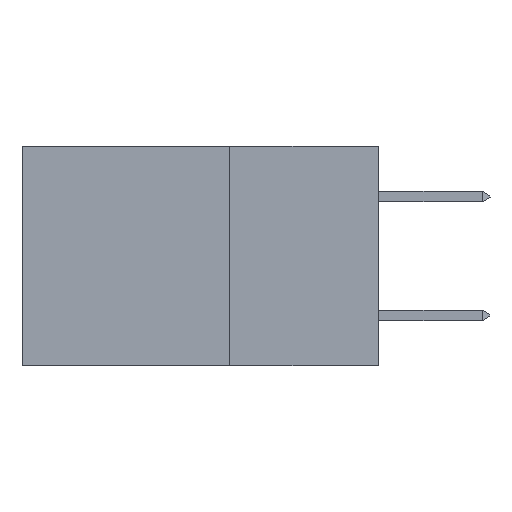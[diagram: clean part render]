
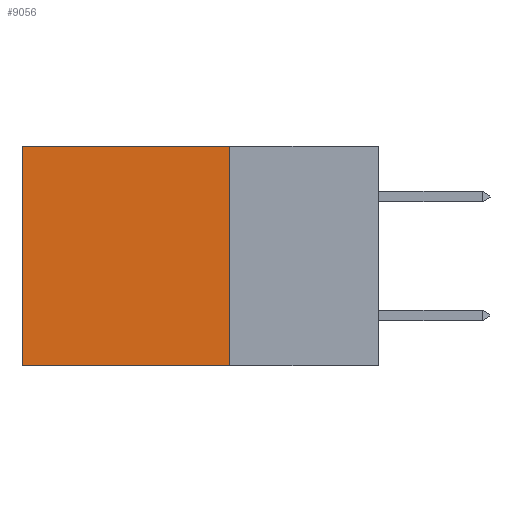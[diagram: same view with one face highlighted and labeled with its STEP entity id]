
A CAD part, left-side view. The second image highlights one B-rep face of the part: STEP entity #9056.
In plain terms, the highlighted planar face has unit normal (-1, 0, 0).
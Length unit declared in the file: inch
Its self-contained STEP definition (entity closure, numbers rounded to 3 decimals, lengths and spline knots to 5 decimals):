
#375 = VERTEX_POINT ( 'NONE', #10993 ) ;
#681 = FACE_OUTER_BOUND ( 'NONE', #2294, .T. ) ;
#1014 = DIRECTION ( 'NONE',  ( 0., 0., -1. ) ) ;
#1057 = VECTOR ( 'NONE', #5978, 39.37008 ) ;
#1110 = ORIENTED_EDGE ( 'NONE', *, *, #8985, .T. ) ;
#1359 = EDGE_CURVE ( 'NONE', #3511, #13293, #1932, .T. ) ;
#1932 = LINE ( 'NONE', #5883, #13370 ) ;
#2178 = CARTESIAN_POINT ( 'NONE',  ( 0.298, 0.6, 0. ) ) ;
#2294 = EDGE_LOOP ( 'NONE', ( #1110, #9230, #5053, #6256 ) ) ;
#3511 = VERTEX_POINT ( 'NONE', #7543 ) ;
#3618 = DIRECTION ( 'NONE',  ( 0., 1., 0. ) ) ;
#5053 = ORIENTED_EDGE ( 'NONE', *, *, #6293, .F. ) ;
#5085 = AXIS2_PLACEMENT_3D ( 'NONE', #14174, #11958, #6084 ) ;
#5883 = CARTESIAN_POINT ( 'NONE',  ( 0.298, 0.25, 0. ) ) ;
#5978 = DIRECTION ( 'NONE',  ( 0., 0., -1. ) ) ;
#6017 = DIRECTION ( 'NONE',  ( 0., 1., 0. ) ) ;
#6084 = DIRECTION ( 'NONE',  ( 0., 0., -1. ) ) ;
#6256 = ORIENTED_EDGE ( 'NONE', *, *, #1359, .T. ) ;
#6293 = EDGE_CURVE ( 'NONE', #3511, #375, #9834, .T. ) ;
#7166 = CARTESIAN_POINT ( 'NONE',  ( 0.298, 0.25, -0.37 ) ) ;
#7177 = PLANE ( 'NONE',  #5085 ) ;
#7543 = CARTESIAN_POINT ( 'NONE',  ( 0.298, 0.25, 0. ) ) ;
#7818 = CARTESIAN_POINT ( 'NONE',  ( 0.298, 0.6, 0. ) ) ;
#8434 = VECTOR ( 'NONE', #6017, 39.37008 ) ;
#8985 = EDGE_CURVE ( 'NONE', #13293, #10444, #11920, .T. ) ;
#9056 = ADVANCED_FACE ( 'NONE', ( #681 ), #7177, .F. ) ;
#9230 = ORIENTED_EDGE ( 'NONE', *, *, #14295, .F. ) ;
#9518 = CARTESIAN_POINT ( 'NONE',  ( 0.298, 0.6, -0.37 ) ) ;
#9834 = LINE ( 'NONE', #15195, #14963 ) ;
#10444 = VERTEX_POINT ( 'NONE', #9518 ) ;
#10993 = CARTESIAN_POINT ( 'NONE',  ( 0.298, 0.25, -0.37 ) ) ;
#11393 = LINE ( 'NONE', #7166, #8434 ) ;
#11920 = LINE ( 'NONE', #2178, #1057 ) ;
#11958 = DIRECTION ( 'NONE',  ( 1., 0., 0. ) ) ;
#13293 = VERTEX_POINT ( 'NONE', #7818 ) ;
#13370 = VECTOR ( 'NONE', #3618, 39.37008 ) ;
#14174 = CARTESIAN_POINT ( 'NONE',  ( 0.298, 0.25, 0. ) ) ;
#14295 = EDGE_CURVE ( 'NONE', #375, #10444, #11393, .T. ) ;
#14963 = VECTOR ( 'NONE', #1014, 39.37008 ) ;
#15195 = CARTESIAN_POINT ( 'NONE',  ( 0.298, 0.25, 0. ) ) ;
